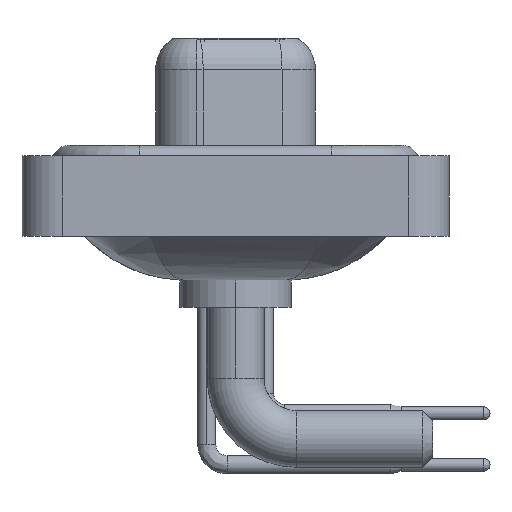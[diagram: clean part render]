
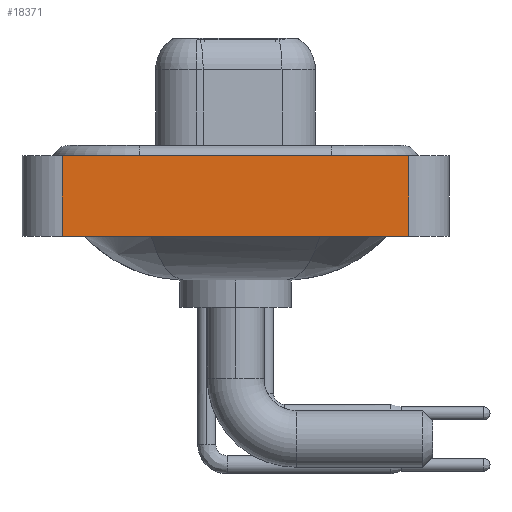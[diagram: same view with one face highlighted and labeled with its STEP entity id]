
A CAD part, left-side view. The second image highlights one B-rep face of the part: STEP entity #18371.
In plain terms, the highlighted planar face has unit normal (-1, 0, 0).
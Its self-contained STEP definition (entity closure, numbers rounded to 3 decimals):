
#447 = EDGE_CURVE ( 'NONE', #9178, #13563, #5723, .T. ) ;
#459 = ORIENTED_EDGE ( 'NONE', *, *, #9956, .F. ) ;
#2207 = CARTESIAN_POINT ( 'NONE',  ( -7.3, -8.55, -3.6 ) ) ;
#2485 = CARTESIAN_POINT ( 'NONE',  ( -7.3, -8.55, 0.4 ) ) ;
#2961 = EDGE_CURVE ( 'NONE', #13563, #11713, #10099, .T. ) ;
#4088 = AXIS2_PLACEMENT_3D ( 'NONE', #8835, #20247, #13510 ) ;
#4281 = CARTESIAN_POINT ( 'NONE',  ( -7.3, -8.55, 0.4 ) ) ;
#4509 = VECTOR ( 'NONE', #5621, 1000. ) ;
#4559 = CARTESIAN_POINT ( 'NONE',  ( -7.3, -8.55, -3.6 ) ) ;
#4579 = LINE ( 'NONE', #12328, #7029 ) ;
#4893 = DIRECTION ( 'NONE',  ( 0., 0., 1. ) ) ;
#5621 = DIRECTION ( 'NONE',  ( 0., -1., 0. ) ) ;
#5723 = LINE ( 'NONE', #19611, #7606 ) ;
#6086 = VECTOR ( 'NONE', #8542, 1000. ) ;
#7029 = VECTOR ( 'NONE', #4893, 1000. ) ;
#7606 = VECTOR ( 'NONE', #16722, 1000. ) ;
#7622 = ORIENTED_EDGE ( 'NONE', *, *, #2961, .T. ) ;
#8542 = DIRECTION ( 'NONE',  ( 0., 0., 1. ) ) ;
#8835 = CARTESIAN_POINT ( 'NONE',  ( -7.3, -8.55, -3.6 ) ) ;
#8914 = VERTEX_POINT ( 'NONE', #11299 ) ;
#9178 = VERTEX_POINT ( 'NONE', #17316 ) ;
#9956 = EDGE_CURVE ( 'NONE', #8914, #11713, #19908, .T. ) ;
#10099 = LINE ( 'NONE', #2207, #6086 ) ;
#11299 = CARTESIAN_POINT ( 'NONE',  ( -7.3, 8.55, 0.4 ) ) ;
#11634 = ORIENTED_EDGE ( 'NONE', *, *, #15611, .F. ) ;
#11680 = EDGE_LOOP ( 'NONE', ( #7622, #459, #11634, #14264 ) ) ;
#11713 = VERTEX_POINT ( 'NONE', #2485 ) ;
#12328 = CARTESIAN_POINT ( 'NONE',  ( -7.3, 8.55, -3.6 ) ) ;
#13510 = DIRECTION ( 'NONE',  ( 0., 0., 1. ) ) ;
#13563 = VERTEX_POINT ( 'NONE', #4559 ) ;
#14264 = ORIENTED_EDGE ( 'NONE', *, *, #447, .T. ) ;
#15611 = EDGE_CURVE ( 'NONE', #9178, #8914, #4579, .T. ) ;
#16722 = DIRECTION ( 'NONE',  ( 0., -1., 0. ) ) ;
#16843 = PLANE ( 'NONE',  #4088 ) ;
#17316 = CARTESIAN_POINT ( 'NONE',  ( -7.3, 8.55, -3.6 ) ) ;
#18371 = ADVANCED_FACE ( 'NONE', ( #19938 ), #16843, .T. ) ;
#19611 = CARTESIAN_POINT ( 'NONE',  ( -7.3, -8.55, -3.6 ) ) ;
#19908 = LINE ( 'NONE', #4281, #4509 ) ;
#19938 = FACE_OUTER_BOUND ( 'NONE', #11680, .T. ) ;
#20247 = DIRECTION ( 'NONE',  ( -1., 0., 0. ) ) ;
